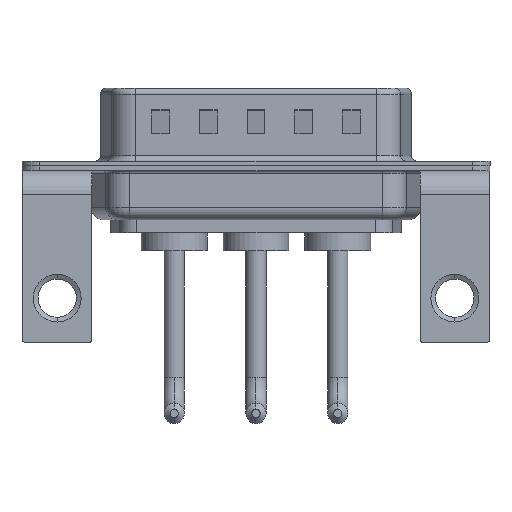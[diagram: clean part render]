
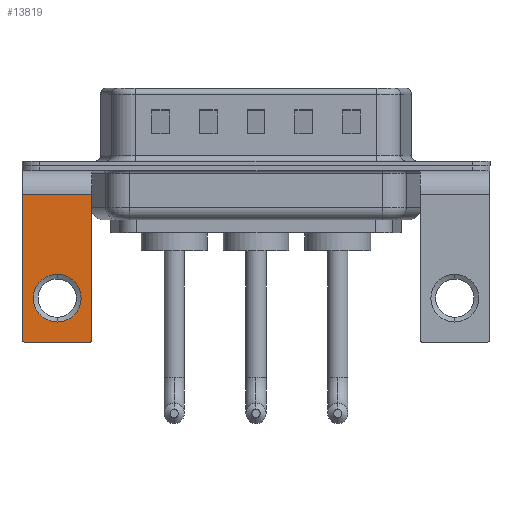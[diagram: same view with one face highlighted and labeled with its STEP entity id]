
A CAD part, front view. The second image highlights one B-rep face of the part: STEP entity #13819.
In plain terms, the highlighted planar face has unit normal (0, -1, 0).
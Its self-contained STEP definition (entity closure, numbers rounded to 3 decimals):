
#48 = EDGE_CURVE ( 'NONE', #7678, #9009, #219, .T. ) ;
#65 = CARTESIAN_POINT ( 'NONE',  ( 0., -6.25, -13.07 ) ) ;
#219 = CIRCLE ( 'NONE', #4506, 0.25 ) ;
#274 = AXIS2_PLACEMENT_3D ( 'NONE', #1785, #10866, #3124 ) ;
#277 = DIRECTION ( 'NONE',  ( 0., 0., 1. ) ) ;
#556 = CIRCLE ( 'NONE', #274, 0.25 ) ;
#1086 = VECTOR ( 'NONE', #9643, 1000. ) ;
#1500 = VECTOR ( 'NONE', #14510, 1000. ) ;
#1785 = CARTESIAN_POINT ( 'NONE',  ( 2.65, -6.25, -14.55 ) ) ;
#1925 = CARTESIAN_POINT ( 'NONE',  ( 2.9, -6.25, -2.4 ) ) ;
#2047 = EDGE_CURVE ( 'NONE', #7821, #10525, #5645, .T. ) ;
#2312 = DIRECTION ( 'NONE',  ( 0., 0., 1. ) ) ;
#2634 = CARTESIAN_POINT ( 'NONE',  ( 2.9, -6.25, -2.4 ) ) ;
#2890 = EDGE_CURVE ( 'NONE', #14466, #9009, #5750, .T. ) ;
#2945 = CARTESIAN_POINT ( 'NONE',  ( 2.65, -6.25, -14.8 ) ) ;
#3124 = DIRECTION ( 'NONE',  ( 0., 0., 1. ) ) ;
#3974 = DIRECTION ( 'NONE',  ( 0., 1., 0. ) ) ;
#4174 = VERTEX_POINT ( 'NONE', #14646 ) ;
#4287 = EDGE_CURVE ( 'NONE', #4174, #7678, #5033, .T. ) ;
#4426 = ORIENTED_EDGE ( 'NONE', *, *, #11490, .T. ) ;
#4506 = AXIS2_PLACEMENT_3D ( 'NONE', #6362, #10172, #10248 ) ;
#4735 = LINE ( 'NONE', #11282, #9089 ) ;
#5033 = LINE ( 'NONE', #11410, #6273 ) ;
#5091 = EDGE_CURVE ( 'NONE', #9919, #8095, #11804, .T. ) ;
#5206 = CARTESIAN_POINT ( 'NONE',  ( 0., -6.25, -11.07 ) ) ;
#5618 = CARTESIAN_POINT ( 'NONE',  ( -2.65, -6.25, -14.8 ) ) ;
#5645 = LINE ( 'NONE', #13276, #1500 ) ;
#5750 = LINE ( 'NONE', #16110, #1086 ) ;
#6132 = ORIENTED_EDGE ( 'NONE', *, *, #48, .T. ) ;
#6273 = VECTOR ( 'NONE', #6367, 1000. ) ;
#6362 = CARTESIAN_POINT ( 'NONE',  ( -2.65, -6.25, -14.55 ) ) ;
#6367 = DIRECTION ( 'NONE',  ( 0., 0., -1. ) ) ;
#6400 = FACE_BOUND ( 'NONE', #8238, .T. ) ;
#7678 = VERTEX_POINT ( 'NONE', #10350 ) ;
#7821 = VERTEX_POINT ( 'NONE', #1925 ) ;
#7945 = DIRECTION ( 'NONE',  ( 0., 1., 0. ) ) ;
#8095 = VERTEX_POINT ( 'NONE', #65 ) ;
#8238 = EDGE_LOOP ( 'NONE', ( #12649, #10950 ) ) ;
#8581 = CARTESIAN_POINT ( 'NONE',  ( 0., -6.25, -11.07 ) ) ;
#9009 = VERTEX_POINT ( 'NONE', #5618 ) ;
#9088 = ORIENTED_EDGE ( 'NONE', *, *, #2890, .F. ) ;
#9089 = VECTOR ( 'NONE', #16104, 1000. ) ;
#9302 = PLANE ( 'NONE',  #11771 ) ;
#9317 = ORIENTED_EDGE ( 'NONE', *, *, #11831, .T. ) ;
#9374 = CARTESIAN_POINT ( 'NONE',  ( 2.9, -6.25, -14.55 ) ) ;
#9643 = DIRECTION ( 'NONE',  ( -1., 0., 0. ) ) ;
#9919 = VERTEX_POINT ( 'NONE', #14363 ) ;
#10113 = DIRECTION ( 'NONE',  ( 0., 0., 1. ) ) ;
#10172 = DIRECTION ( 'NONE',  ( 0., -1., 0. ) ) ;
#10248 = DIRECTION ( 'NONE',  ( 0., 0., 1. ) ) ;
#10350 = CARTESIAN_POINT ( 'NONE',  ( -2.9, -6.25, -14.55 ) ) ;
#10525 = VERTEX_POINT ( 'NONE', #9374 ) ;
#10866 = DIRECTION ( 'NONE',  ( 0., -1., 0. ) ) ;
#10881 = ORIENTED_EDGE ( 'NONE', *, *, #4287, .T. ) ;
#10950 = ORIENTED_EDGE ( 'NONE', *, *, #5091, .T. ) ;
#11282 = CARTESIAN_POINT ( 'NONE',  ( 2.9, -6.25, -2.4 ) ) ;
#11410 = CARTESIAN_POINT ( 'NONE',  ( -2.9, -6.25, -2.4 ) ) ;
#11490 = EDGE_CURVE ( 'NONE', #7821, #4174, #4735, .T. ) ;
#11771 = AXIS2_PLACEMENT_3D ( 'NONE', #2634, #3974, #277 ) ;
#11804 = CIRCLE ( 'NONE', #12609, 2. ) ;
#11831 = EDGE_CURVE ( 'NONE', #14466, #10525, #556, .T. ) ;
#12137 = EDGE_CURVE ( 'NONE', #8095, #9919, #15460, .T. ) ;
#12609 = AXIS2_PLACEMENT_3D ( 'NONE', #8581, #14955, #2312 ) ;
#12649 = ORIENTED_EDGE ( 'NONE', *, *, #12137, .T. ) ;
#12734 = ORIENTED_EDGE ( 'NONE', *, *, #2047, .F. ) ;
#13276 = CARTESIAN_POINT ( 'NONE',  ( 2.9, -6.25, -2.4 ) ) ;
#13600 = AXIS2_PLACEMENT_3D ( 'NONE', #5206, #7945, #10113 ) ;
#13819 = ADVANCED_FACE ( 'NONE', ( #6400, #15272 ), #9302, .F. ) ;
#13974 = EDGE_LOOP ( 'NONE', ( #10881, #6132, #9088, #9317, #12734, #4426 ) ) ;
#14363 = CARTESIAN_POINT ( 'NONE',  ( 0., -6.25, -9.07 ) ) ;
#14466 = VERTEX_POINT ( 'NONE', #2945 ) ;
#14510 = DIRECTION ( 'NONE',  ( 0., 0., -1. ) ) ;
#14646 = CARTESIAN_POINT ( 'NONE',  ( -2.9, -6.25, -2.4 ) ) ;
#14955 = DIRECTION ( 'NONE',  ( 0., 1., 0. ) ) ;
#15272 = FACE_OUTER_BOUND ( 'NONE', #13974, .T. ) ;
#15460 = CIRCLE ( 'NONE', #13600, 2. ) ;
#16104 = DIRECTION ( 'NONE',  ( -1., 0., 0. ) ) ;
#16110 = CARTESIAN_POINT ( 'NONE',  ( 2.9, -6.25, -14.8 ) ) ;
